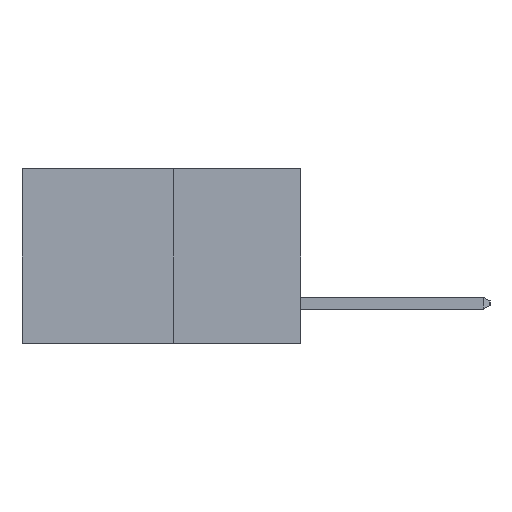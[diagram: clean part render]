
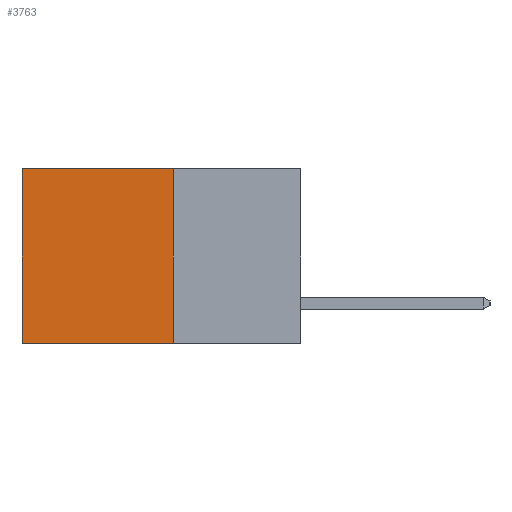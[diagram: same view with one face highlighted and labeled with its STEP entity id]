
A CAD part, left-side view. The second image highlights one B-rep face of the part: STEP entity #3763.
In plain terms, the highlighted planar face has unit normal (-1, 0, 0).
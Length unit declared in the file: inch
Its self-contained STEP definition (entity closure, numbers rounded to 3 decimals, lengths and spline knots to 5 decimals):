
#327 = LINE ( 'NONE', #15911, #8758 ) ;
#533 = ORIENTED_EDGE ( 'NONE', *, *, #12674, .T. ) ;
#686 = CARTESIAN_POINT ( 'NONE',  ( 0.277, 0.27, -0.37 ) ) ;
#1200 = CARTESIAN_POINT ( 'NONE',  ( 0.277, 0.27, -0.37 ) ) ;
#2416 = EDGE_CURVE ( 'NONE', #8538, #7724, #8368, .T. ) ;
#3524 = VERTEX_POINT ( 'NONE', #11636 ) ;
#3763 = ADVANCED_FACE ( 'NONE', ( #7280 ), #4704, .F. ) ;
#4704 = PLANE ( 'NONE',  #14316 ) ;
#5806 = CARTESIAN_POINT ( 'NONE',  ( 0.277, 0.59, 0. ) ) ;
#6557 = ORIENTED_EDGE ( 'NONE', *, *, #17068, .T. ) ;
#7222 = DIRECTION ( 'NONE',  ( 1., 0., 0. ) ) ;
#7280 = FACE_OUTER_BOUND ( 'NONE', #16520, .T. ) ;
#7587 = VECTOR ( 'NONE', #16841, 39.37008 ) ;
#7663 = DIRECTION ( 'NONE',  ( 0., 0., -1. ) ) ;
#7724 = VERTEX_POINT ( 'NONE', #7972 ) ;
#7942 = DIRECTION ( 'NONE',  ( 0., 0., -1. ) ) ;
#7972 = CARTESIAN_POINT ( 'NONE',  ( 0.277, 0.27, -0.37 ) ) ;
#8260 = ORIENTED_EDGE ( 'NONE', *, *, #14789, .F. ) ;
#8368 = LINE ( 'NONE', #1200, #11497 ) ;
#8538 = VERTEX_POINT ( 'NONE', #14779 ) ;
#8758 = VECTOR ( 'NONE', #17059, 39.37008 ) ;
#9265 = CARTESIAN_POINT ( 'NONE',  ( 0.277, 0.27, 0. ) ) ;
#11144 = LINE ( 'NONE', #9265, #7587 ) ;
#11497 = VECTOR ( 'NONE', #7663, 39.37008 ) ;
#11636 = CARTESIAN_POINT ( 'NONE',  ( 0.277, 0.59, -0.37 ) ) ;
#12674 = EDGE_CURVE ( 'NONE', #8538, #15945, #11144, .T. ) ;
#13940 = ORIENTED_EDGE ( 'NONE', *, *, #2416, .F. ) ;
#14315 = DIRECTION ( 'NONE',  ( 0., 0., -1. ) ) ;
#14316 = AXIS2_PLACEMENT_3D ( 'NONE', #686, #7222, #14315 ) ;
#14779 = CARTESIAN_POINT ( 'NONE',  ( 0.277, 0.27, 0. ) ) ;
#14789 = EDGE_CURVE ( 'NONE', #7724, #3524, #327, .T. ) ;
#15911 = CARTESIAN_POINT ( 'NONE',  ( 0.277, 0.27, -0.37 ) ) ;
#15945 = VERTEX_POINT ( 'NONE', #5806 ) ;
#16046 = LINE ( 'NONE', #16859, #16414 ) ;
#16414 = VECTOR ( 'NONE', #7942, 39.37008 ) ;
#16520 = EDGE_LOOP ( 'NONE', ( #6557, #8260, #13940, #533 ) ) ;
#16841 = DIRECTION ( 'NONE',  ( 0., 1., 0. ) ) ;
#16859 = CARTESIAN_POINT ( 'NONE',  ( 0.277, 0.59, -0.37 ) ) ;
#17059 = DIRECTION ( 'NONE',  ( 0., 1., 0. ) ) ;
#17068 = EDGE_CURVE ( 'NONE', #15945, #3524, #16046, .T. ) ;
